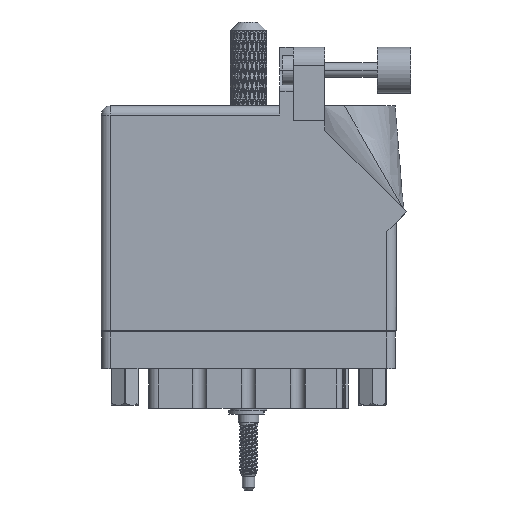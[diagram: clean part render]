
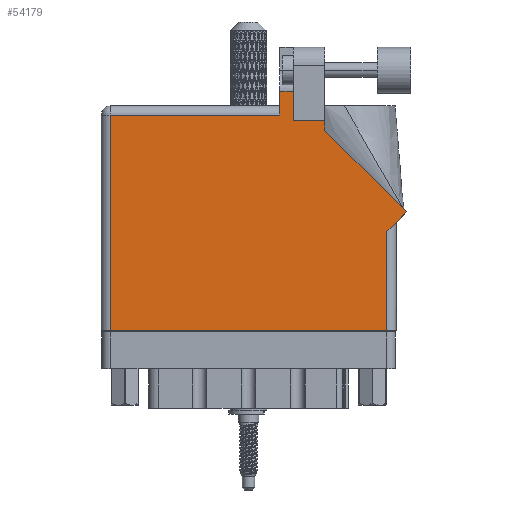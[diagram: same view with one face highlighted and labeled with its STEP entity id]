
A CAD part, front view. The second image highlights one B-rep face of the part: STEP entity #54179.
In plain terms, the highlighted face is planar.
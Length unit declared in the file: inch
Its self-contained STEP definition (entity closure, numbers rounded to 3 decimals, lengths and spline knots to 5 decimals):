
#129 = FACE_OUTER_BOUND ( 'NONE', #11086, .T. ) ;
#202 = DIRECTION ( 'NONE',  ( -0.707, 0.707, 0. ) ) ;
#1347 = VECTOR ( 'NONE', #70441, 39.37008 ) ;
#1868 = CARTESIAN_POINT ( 'NONE',  ( 1.524, 1.36442, 0. ) ) ;
#5106 = EDGE_CURVE ( 'NONE', #15922, #21633, #113925, .T. ) ;
#6263 = VECTOR ( 'NONE', #77322, 39.37008 ) ;
#7558 = EDGE_CURVE ( 'NONE', #76615, #85290, #68755, .T. ) ;
#8415 = ORIENTED_EDGE ( 'NONE', *, *, #101811, .T. ) ;
#9030 = CARTESIAN_POINT ( 'NONE',  ( 1.217, 1.6315, 0. ) ) ;
#9068 = CARTESIAN_POINT ( 'NONE',  ( 1.311, 1.43, 0. ) ) ;
#9443 = VERTEX_POINT ( 'NONE', #9030 ) ;
#9818 = AXIS2_PLACEMENT_3D ( 'NONE', #27525, #18511, #81508 ) ;
#11086 = EDGE_LOOP ( 'NONE', ( #8415, #32433, #20397, #51294, #63502, #12154, #17050, #40929, #28179, #75841, #39913 ) ) ;
#11103 = CARTESIAN_POINT ( 'NONE',  ( 0.062, 0., 0. ) ) ;
#11526 = LINE ( 'NONE', #98139, #85738 ) ;
#12154 = ORIENTED_EDGE ( 'NONE', *, *, #7558, .T. ) ;
#15922 = VERTEX_POINT ( 'NONE', #37990 ) ;
#16721 = VERTEX_POINT ( 'NONE', #34246 ) ;
#17050 = ORIENTED_EDGE ( 'NONE', *, *, #40339, .T. ) ;
#17962 = CARTESIAN_POINT ( 'NONE',  ( 1.64177, 1.6315, 0. ) ) ;
#18511 = DIRECTION ( 'NONE',  ( 0., 0., -1. ) ) ;
#19859 = VERTEX_POINT ( 'NONE', #38038 ) ;
#20207 = DIRECTION ( 'NONE',  ( 1., 0., 0. ) ) ;
#20397 = ORIENTED_EDGE ( 'NONE', *, *, #40031, .T. ) ;
#21633 = VERTEX_POINT ( 'NONE', #75597 ) ;
#23700 = LINE ( 'NONE', #97109, #1347 ) ;
#27525 = CARTESIAN_POINT ( 'NONE',  ( 0., 1.53, 0. ) ) ;
#28179 = ORIENTED_EDGE ( 'NONE', *, *, #100126, .T. ) ;
#31478 = LINE ( 'NONE', #71732, #97336 ) ;
#32433 = ORIENTED_EDGE ( 'NONE', *, *, #33549, .T. ) ;
#33549 = EDGE_CURVE ( 'NONE', #36495, #9443, #59587, .T. ) ;
#34246 = CARTESIAN_POINT ( 'NONE',  ( 1.948, 0.675, 0. ) ) ;
#36495 = VERTEX_POINT ( 'NONE', #112231 ) ;
#37990 = CARTESIAN_POINT ( 'NONE',  ( 1.524, 1.36442, 0. ) ) ;
#38038 = CARTESIAN_POINT ( 'NONE',  ( 2.08071, 0.80771, 0. ) ) ;
#38156 = CARTESIAN_POINT ( 'NONE',  ( 1.217, 1.468, 0. ) ) ;
#39913 = ORIENTED_EDGE ( 'NONE', *, *, #102612, .T. ) ;
#40031 = EDGE_CURVE ( 'NONE', #9443, #55760, #70658, .T. ) ;
#40339 = EDGE_CURVE ( 'NONE', #85290, #16721, #69201, .T. ) ;
#40929 = ORIENTED_EDGE ( 'NONE', *, *, #46692, .T. ) ;
#43850 = VECTOR ( 'NONE', #47422, 39.37008 ) ;
#45411 = VECTOR ( 'NONE', #77451, 39.37008 ) ;
#45928 = LINE ( 'NONE', #113962, #111791 ) ;
#46535 = LINE ( 'NONE', #110612, #105430 ) ;
#46692 = EDGE_CURVE ( 'NONE', #16721, #19859, #23700, .T. ) ;
#47422 = DIRECTION ( 'NONE',  ( 0., 1., 0. ) ) ;
#48407 = VECTOR ( 'NONE', #61790, 39.37008 ) ;
#49625 = VERTEX_POINT ( 'NONE', #9068 ) ;
#50854 = LINE ( 'NONE', #101069, #43850 ) ;
#51294 = ORIENTED_EDGE ( 'NONE', *, *, #79003, .T. ) ;
#54179 = ADVANCED_FACE ( 'NONE', ( #129 ), #115985, .F. ) ;
#55744 = CARTESIAN_POINT ( 'NONE',  ( 0.062, 1.468, 0. ) ) ;
#55760 = VERTEX_POINT ( 'NONE', #38156 ) ;
#55793 = VERTEX_POINT ( 'NONE', #55744 ) ;
#59587 = LINE ( 'NONE', #17962, #48407 ) ;
#61790 = DIRECTION ( 'NONE',  ( -1., 0., 0. ) ) ;
#63456 = VECTOR ( 'NONE', #91444, 39.37008 ) ;
#63502 = ORIENTED_EDGE ( 'NONE', *, *, #83792, .T. ) ;
#65923 = CARTESIAN_POINT ( 'NONE',  ( 0., 0., 0. ) ) ;
#68755 = LINE ( 'NONE', #65923, #103837 ) ;
#69201 = LINE ( 'NONE', #112581, #6263 ) ;
#69291 = DIRECTION ( 'NONE',  ( 0., -1., 0. ) ) ;
#70441 = DIRECTION ( 'NONE',  ( 0.707, 0.707, 0. ) ) ;
#70658 = LINE ( 'NONE', #95475, #45411 ) ;
#71732 = CARTESIAN_POINT ( 'NONE',  ( 2.08071, 0.80771, 0. ) ) ;
#75597 = CARTESIAN_POINT ( 'NONE',  ( 1.524, 1.43, 0. ) ) ;
#75841 = ORIENTED_EDGE ( 'NONE', *, *, #5106, .T. ) ;
#76615 = VERTEX_POINT ( 'NONE', #11103 ) ;
#77322 = DIRECTION ( 'NONE',  ( 0., 1., 0. ) ) ;
#77451 = DIRECTION ( 'NONE',  ( 0., -1., 0. ) ) ;
#79003 = EDGE_CURVE ( 'NONE', #55760, #55793, #11526, .T. ) ;
#81508 = DIRECTION ( 'NONE',  ( -1., 0., 0. ) ) ;
#82411 = DIRECTION ( 'NONE',  ( -1., 0., 0. ) ) ;
#83792 = EDGE_CURVE ( 'NONE', #55793, #76615, #45928, .T. ) ;
#85290 = VERTEX_POINT ( 'NONE', #86076 ) ;
#85738 = VECTOR ( 'NONE', #88735, 39.37008 ) ;
#86076 = CARTESIAN_POINT ( 'NONE',  ( 1.948, 0., 0. ) ) ;
#88735 = DIRECTION ( 'NONE',  ( -1., 0., 0. ) ) ;
#91444 = DIRECTION ( 'NONE',  ( 0., 1., 0. ) ) ;
#95475 = CARTESIAN_POINT ( 'NONE',  ( 1.217, 1.53, 0. ) ) ;
#97109 = CARTESIAN_POINT ( 'NONE',  ( 2.01, 0.737, 0. ) ) ;
#97336 = VECTOR ( 'NONE', #202, 39.37008 ) ;
#98139 = CARTESIAN_POINT ( 'NONE',  ( 0., 1.468, 0. ) ) ;
#100126 = EDGE_CURVE ( 'NONE', #19859, #15922, #31478, .T. ) ;
#101069 = CARTESIAN_POINT ( 'NONE',  ( 1.311, 1.43, 0. ) ) ;
#101811 = EDGE_CURVE ( 'NONE', #49625, #36495, #50854, .T. ) ;
#102612 = EDGE_CURVE ( 'NONE', #21633, #49625, #46535, .T. ) ;
#103837 = VECTOR ( 'NONE', #20207, 39.37008 ) ;
#105430 = VECTOR ( 'NONE', #82411, 39.37008 ) ;
#110612 = CARTESIAN_POINT ( 'NONE',  ( 1.524, 1.43, 0. ) ) ;
#111791 = VECTOR ( 'NONE', #69291, 39.37008 ) ;
#112231 = CARTESIAN_POINT ( 'NONE',  ( 1.311, 1.6315, 0. ) ) ;
#112581 = CARTESIAN_POINT ( 'NONE',  ( 1.948, 0.737, 0. ) ) ;
#113925 = LINE ( 'NONE', #1868, #63456 ) ;
#113962 = CARTESIAN_POINT ( 'NONE',  ( 0.062, 0., 0. ) ) ;
#115985 = PLANE ( 'NONE',  #9818 ) ;
